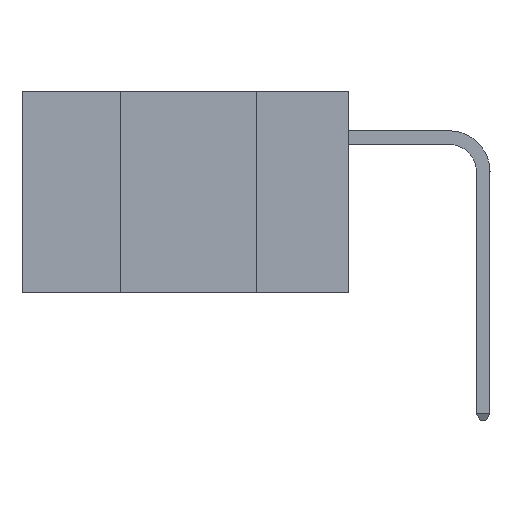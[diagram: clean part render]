
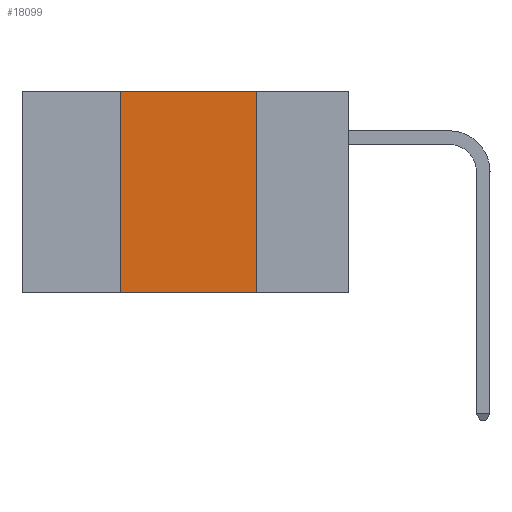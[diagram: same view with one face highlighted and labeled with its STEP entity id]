
A CAD part, left-side view. The second image highlights one B-rep face of the part: STEP entity #18099.
In plain terms, the highlighted planar face has unit normal (-1, 0, 0).
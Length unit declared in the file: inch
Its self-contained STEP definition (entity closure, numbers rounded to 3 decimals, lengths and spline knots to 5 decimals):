
#445 = EDGE_CURVE ( 'NONE', #1094, #22082, #10679, .T. ) ;
#843 = ORIENTED_EDGE ( 'NONE', *, *, #25637, .T. ) ;
#1094 = VERTEX_POINT ( 'NONE', #18218 ) ;
#1305 = DIRECTION ( 'NONE',  ( 1., 0., 0. ) ) ;
#3621 = EDGE_CURVE ( 'NONE', #22082, #29359, #11077, .T. ) ;
#3811 = LINE ( 'NONE', #26829, #26846 ) ;
#8271 = CARTESIAN_POINT ( 'NONE',  ( 0., 0.42, 0. ) ) ;
#9363 = VECTOR ( 'NONE', #33284, 39.37008 ) ;
#10636 = CARTESIAN_POINT ( 'NONE',  ( 0., 0.6, 0. ) ) ;
#10679 = LINE ( 'NONE', #11695, #25370 ) ;
#11077 = LINE ( 'NONE', #23502, #26757 ) ;
#11222 = DIRECTION ( 'NONE',  ( 0., -1., 0. ) ) ;
#11695 = CARTESIAN_POINT ( 'NONE',  ( 0., 0.6, 0. ) ) ;
#12252 = CARTESIAN_POINT ( 'NONE',  ( 0., 0.42, -0.37 ) ) ;
#18099 = ADVANCED_FACE ( 'NONE', ( #35234 ), #20079, .F. ) ;
#18218 = CARTESIAN_POINT ( 'NONE',  ( 0., 0.42, 0. ) ) ;
#20079 = PLANE ( 'NONE',  #28272 ) ;
#20221 = CARTESIAN_POINT ( 'NONE',  ( 0., 0.17, 0. ) ) ;
#20477 = DIRECTION ( 'NONE',  ( 0., 0., -1. ) ) ;
#21415 = ORIENTED_EDGE ( 'NONE', *, *, #445, .F. ) ;
#22082 = VERTEX_POINT ( 'NONE', #20221 ) ;
#23240 = DIRECTION ( 'NONE',  ( 0., 0., -1. ) ) ;
#23502 = CARTESIAN_POINT ( 'NONE',  ( 0., 0.17, 0. ) ) ;
#25370 = VECTOR ( 'NONE', #30413, 39.37008 ) ;
#25637 = EDGE_CURVE ( 'NONE', #28227, #29359, #3811, .T. ) ;
#26757 = VECTOR ( 'NONE', #20477, 39.37008 ) ;
#26829 = CARTESIAN_POINT ( 'NONE',  ( 0., 0.6, -0.37 ) ) ;
#26846 = VECTOR ( 'NONE', #11222, 39.37008 ) ;
#28227 = VERTEX_POINT ( 'NONE', #12252 ) ;
#28272 = AXIS2_PLACEMENT_3D ( 'NONE', #10636, #1305, #23240 ) ;
#29359 = VERTEX_POINT ( 'NONE', #35321 ) ;
#29584 = EDGE_CURVE ( 'NONE', #28227, #1094, #34302, .T. ) ;
#30192 = ORIENTED_EDGE ( 'NONE', *, *, #3621, .F. ) ;
#30413 = DIRECTION ( 'NONE',  ( 0., -1., 0. ) ) ;
#31677 = ORIENTED_EDGE ( 'NONE', *, *, #29584, .F. ) ;
#33284 = DIRECTION ( 'NONE',  ( 0., 0., 1. ) ) ;
#34302 = LINE ( 'NONE', #8271, #9363 ) ;
#35234 = FACE_OUTER_BOUND ( 'NONE', #35727, .T. ) ;
#35321 = CARTESIAN_POINT ( 'NONE',  ( 0., 0.17, -0.37 ) ) ;
#35727 = EDGE_LOOP ( 'NONE', ( #30192, #21415, #31677, #843 ) ) ;
